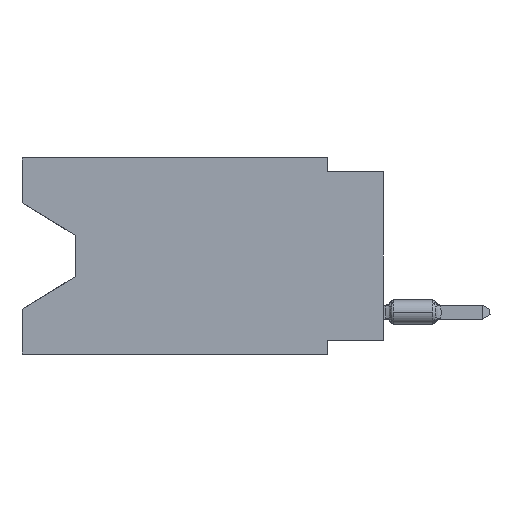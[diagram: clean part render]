
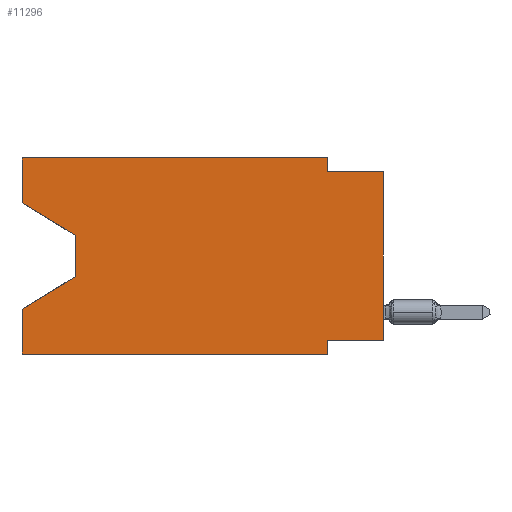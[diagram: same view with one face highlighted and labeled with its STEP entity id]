
A CAD part, left-side view. The second image highlights one B-rep face of the part: STEP entity #11296.
In plain terms, the highlighted planar face has unit normal (-1, 0, 0).
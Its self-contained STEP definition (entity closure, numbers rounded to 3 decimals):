
#57 = VERTEX_POINT ( 'NONE', #39566 ) ;
#108 = EDGE_LOOP ( 'NONE', ( #8144, #22684, #30498, #50662, #31186, #41535, #46782, #56925, #32086, #71942, #3606, #16433 ) ) ;
#1068 = PLANE ( 'NONE',  #1968 ) ;
#1968 = AXIS2_PLACEMENT_3D ( 'NONE', #12048, #12398, #63281 ) ;
#2078 = CARTESIAN_POINT ( 'NONE',  ( 0., 0., -0.635 ) ) ;
#2333 = CARTESIAN_POINT ( 'NONE',  ( 0., 16.383, 0. ) ) ;
#2484 = VERTEX_POINT ( 'NONE', #30416 ) ;
#2878 = EDGE_CURVE ( 'NONE', #33343, #67275, #35459, .T. ) ;
#3177 = VERTEX_POINT ( 'NONE', #44569 ) ;
#3424 = CARTESIAN_POINT ( 'NONE',  ( 0., 13.97, -5.385 ) ) ;
#3606 = ORIENTED_EDGE ( 'NONE', *, *, #69623, .F. ) ;
#4021 = VECTOR ( 'NONE', #53665, 1000. ) ;
#5123 = VERTEX_POINT ( 'NONE', #53249 ) ;
#5125 = LINE ( 'NONE', #50864, #36208 ) ;
#5552 = VECTOR ( 'NONE', #8702, 1000. ) ;
#6332 = CARTESIAN_POINT ( 'NONE',  ( 0., 16.383, 0. ) ) ;
#6930 = DIRECTION ( 'NONE',  ( 0., 0., -1. ) ) ;
#8076 = EDGE_CURVE ( 'NONE', #57, #2484, #29756, .T. ) ;
#8144 = ORIENTED_EDGE ( 'NONE', *, *, #61046, .T. ) ;
#8272 = CARTESIAN_POINT ( 'NONE',  ( 0., 0., -8.255 ) ) ;
#8702 = DIRECTION ( 'NONE',  ( 0., 0., 1. ) ) ;
#10605 = DIRECTION ( 'NONE',  ( 0., 0., 1. ) ) ;
#10613 = VERTEX_POINT ( 'NONE', #3424 ) ;
#11296 = ADVANCED_FACE ( 'NONE', ( #12752 ), #1068, .F. ) ;
#11308 = CARTESIAN_POINT ( 'NONE',  ( 0., 2.54, -8.255 ) ) ;
#11601 = VECTOR ( 'NONE', #37888, 1000. ) ;
#12048 = CARTESIAN_POINT ( 'NONE',  ( 0., 16.383, 0. ) ) ;
#12224 = DIRECTION ( 'NONE',  ( 0., 0., 1. ) ) ;
#12398 = DIRECTION ( 'NONE',  ( 1., 0., 0. ) ) ;
#12567 = VECTOR ( 'NONE', #50635, 1000. ) ;
#12752 = FACE_OUTER_BOUND ( 'NONE', #108, .T. ) ;
#14070 = CARTESIAN_POINT ( 'NONE',  ( 0., 16.383, -8.89 ) ) ;
#16433 = ORIENTED_EDGE ( 'NONE', *, *, #40796, .F. ) ;
#16551 = VERTEX_POINT ( 'NONE', #66897 ) ;
#17020 = VECTOR ( 'NONE', #57241, 1000. ) ;
#17740 = EDGE_CURVE ( 'NONE', #58372, #67275, #40833, .T. ) ;
#18506 = DIRECTION ( 'NONE',  ( 0., -1., 0. ) ) ;
#19136 = VECTOR ( 'NONE', #70928, 1000. ) ;
#20398 = CARTESIAN_POINT ( 'NONE',  ( 0., 13.97, -3.505 ) ) ;
#22684 = ORIENTED_EDGE ( 'NONE', *, *, #34335, .T. ) ;
#23280 = CARTESIAN_POINT ( 'NONE',  ( 0., 16.383, -8.89 ) ) ;
#25082 = LINE ( 'NONE', #8272, #4021 ) ;
#26237 = LINE ( 'NONE', #20398, #19136 ) ;
#27235 = EDGE_CURVE ( 'NONE', #28043, #33343, #25082, .T. ) ;
#28043 = VERTEX_POINT ( 'NONE', #42479 ) ;
#29756 = LINE ( 'NONE', #34895, #17020 ) ;
#30416 = CARTESIAN_POINT ( 'NONE',  ( 0., 2.54, -0.635 ) ) ;
#30498 = ORIENTED_EDGE ( 'NONE', *, *, #52470, .T. ) ;
#30718 = CARTESIAN_POINT ( 'NONE',  ( 0., 2.54, -8.89 ) ) ;
#30770 = EDGE_CURVE ( 'NONE', #28043, #62031, #5125, .T. ) ;
#31186 = ORIENTED_EDGE ( 'NONE', *, *, #17740, .T. ) ;
#31210 = LINE ( 'NONE', #71835, #55050 ) ;
#31727 = EDGE_CURVE ( 'NONE', #58372, #16551, #62022, .T. ) ;
#32028 = LINE ( 'NONE', #60586, #11601 ) ;
#32086 = ORIENTED_EDGE ( 'NONE', *, *, #72372, .F. ) ;
#33343 = VERTEX_POINT ( 'NONE', #11308 ) ;
#34335 = EDGE_CURVE ( 'NONE', #5123, #10613, #26237, .T. ) ;
#34895 = CARTESIAN_POINT ( 'NONE',  ( 0., 2.54, 0. ) ) ;
#35459 = LINE ( 'NONE', #64016, #38724 ) ;
#36152 = CARTESIAN_POINT ( 'NONE',  ( 0., 16.383, 0. ) ) ;
#36208 = VECTOR ( 'NONE', #10605, 1000. ) ;
#36516 = LINE ( 'NONE', #36152, #5552 ) ;
#37888 = DIRECTION ( 'NONE',  ( 0., -0.855, -0.519 ) ) ;
#38724 = VECTOR ( 'NONE', #6930, 1000. ) ;
#39566 = CARTESIAN_POINT ( 'NONE',  ( 0., 2.54, 0. ) ) ;
#40796 = EDGE_CURVE ( 'NONE', #3177, #65654, #36516, .T. ) ;
#40833 = LINE ( 'NONE', #23280, #71701 ) ;
#41535 = ORIENTED_EDGE ( 'NONE', *, *, #2878, .F. ) ;
#42479 = CARTESIAN_POINT ( 'NONE',  ( 0., 0., -8.255 ) ) ;
#42559 = DIRECTION ( 'NONE',  ( 0., -1., 0. ) ) ;
#44569 = CARTESIAN_POINT ( 'NONE',  ( 0., 16.383, -2.038 ) ) ;
#46605 = CARTESIAN_POINT ( 'NONE',  ( 0., 13.97, -5.385 ) ) ;
#46782 = ORIENTED_EDGE ( 'NONE', *, *, #27235, .F. ) ;
#47657 = CARTESIAN_POINT ( 'NONE',  ( 0., 16.383, 0. ) ) ;
#48578 = VECTOR ( 'NONE', #68933, 1000. ) ;
#50635 = DIRECTION ( 'NONE',  ( 0., -1., 0. ) ) ;
#50662 = ORIENTED_EDGE ( 'NONE', *, *, #31727, .F. ) ;
#50864 = CARTESIAN_POINT ( 'NONE',  ( 0., 0., 0. ) ) ;
#52058 = LINE ( 'NONE', #6332, #12567 ) ;
#52470 = EDGE_CURVE ( 'NONE', #10613, #16551, #63796, .T. ) ;
#53249 = CARTESIAN_POINT ( 'NONE',  ( 0., 13.97, -3.505 ) ) ;
#53665 = DIRECTION ( 'NONE',  ( 0., 1., 0. ) ) ;
#55050 = VECTOR ( 'NONE', #42559, 1000. ) ;
#56925 = ORIENTED_EDGE ( 'NONE', *, *, #30770, .T. ) ;
#57241 = DIRECTION ( 'NONE',  ( 0., 0., -1. ) ) ;
#58372 = VERTEX_POINT ( 'NONE', #14070 ) ;
#60586 = CARTESIAN_POINT ( 'NONE',  ( 0., 16.383, -2.038 ) ) ;
#61046 = EDGE_CURVE ( 'NONE', #3177, #5123, #32028, .T. ) ;
#62022 = LINE ( 'NONE', #2333, #63165 ) ;
#62031 = VERTEX_POINT ( 'NONE', #2078 ) ;
#63165 = VECTOR ( 'NONE', #12224, 1000. ) ;
#63281 = DIRECTION ( 'NONE',  ( 0., 0., -1. ) ) ;
#63796 = LINE ( 'NONE', #46605, #48578 ) ;
#64016 = CARTESIAN_POINT ( 'NONE',  ( 0., 2.54, -8.89 ) ) ;
#65654 = VERTEX_POINT ( 'NONE', #47657 ) ;
#66897 = CARTESIAN_POINT ( 'NONE',  ( 0., 16.383, -6.852 ) ) ;
#67275 = VERTEX_POINT ( 'NONE', #30718 ) ;
#68933 = DIRECTION ( 'NONE',  ( 0., 0.855, -0.519 ) ) ;
#69623 = EDGE_CURVE ( 'NONE', #65654, #57, #52058, .T. ) ;
#70928 = DIRECTION ( 'NONE',  ( 0., 0., -1. ) ) ;
#71701 = VECTOR ( 'NONE', #18506, 1000. ) ;
#71835 = CARTESIAN_POINT ( 'NONE',  ( 0., 0., -0.635 ) ) ;
#71942 = ORIENTED_EDGE ( 'NONE', *, *, #8076, .F. ) ;
#72372 = EDGE_CURVE ( 'NONE', #2484, #62031, #31210, .T. ) ;
